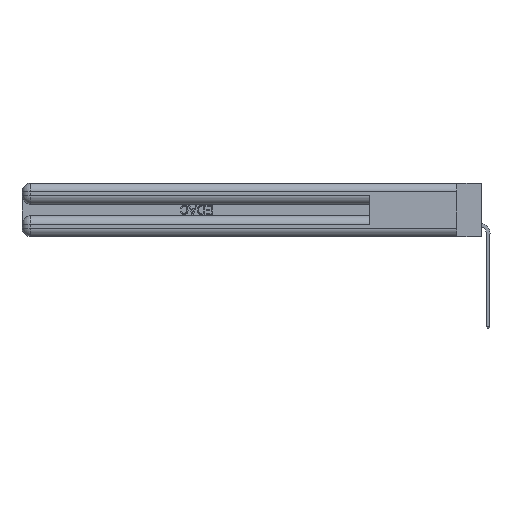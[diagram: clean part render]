
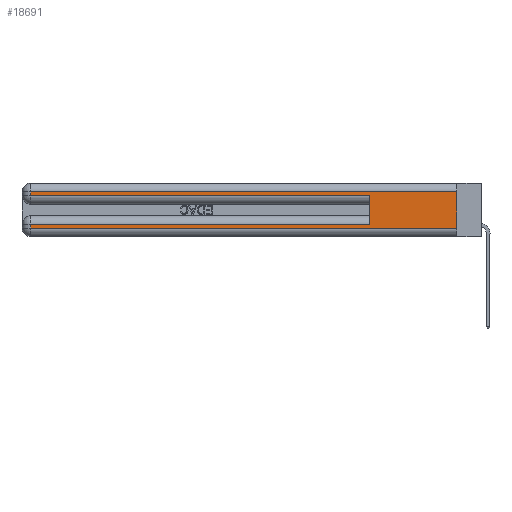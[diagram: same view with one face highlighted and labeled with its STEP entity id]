
A CAD part, left-side view. The second image highlights one B-rep face of the part: STEP entity #18691.
In plain terms, the highlighted planar face has unit normal (-1, 0, 0).
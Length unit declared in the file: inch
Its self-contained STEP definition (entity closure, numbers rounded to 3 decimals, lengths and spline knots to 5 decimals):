
#253 = LINE ( 'NONE', #23787, #23761 ) ;
#607 = CARTESIAN_POINT ( 'NONE',  ( 0., 2.94, 0.285 ) ) ;
#919 = VERTEX_POINT ( 'NONE', #7942 ) ;
#1976 = EDGE_CURVE ( 'NONE', #4796, #17353, #26263, .T. ) ;
#2054 = PLANE ( 'NONE',  #35698 ) ;
#2507 = DIRECTION ( 'NONE',  ( 0., 0., -1. ) ) ;
#3326 = ORIENTED_EDGE ( 'NONE', *, *, #7825, .T. ) ;
#3944 = EDGE_CURVE ( 'NONE', #32960, #919, #253, .T. ) ;
#4224 = LINE ( 'NONE', #21751, #16475 ) ;
#4229 = VERTEX_POINT ( 'NONE', #607 ) ;
#4796 = VERTEX_POINT ( 'NONE', #25364 ) ;
#4893 = DIRECTION ( 'NONE',  ( 0., 1., 0. ) ) ;
#4977 = CARTESIAN_POINT ( 'NONE',  ( 0., 2.94, 0.31 ) ) ;
#5818 = LINE ( 'NONE', #26309, #6734 ) ;
#6442 = FACE_OUTER_BOUND ( 'NONE', #36569, .T. ) ;
#6734 = VECTOR ( 'NONE', #26450, 39.37008 ) ;
#6960 = ORIENTED_EDGE ( 'NONE', *, *, #1976, .T. ) ;
#7302 = EDGE_CURVE ( 'NONE', #8050, #24421, #7932, .T. ) ;
#7433 = LINE ( 'NONE', #16743, #38401 ) ;
#7460 = VECTOR ( 'NONE', #38694, 39.37008 ) ;
#7825 = EDGE_CURVE ( 'NONE', #8050, #9718, #7433, .T. ) ;
#7852 = DIRECTION ( 'NONE',  ( 0., -1., 0. ) ) ;
#7881 = ORIENTED_EDGE ( 'NONE', *, *, #24158, .T. ) ;
#7932 = LINE ( 'NONE', #17477, #25278 ) ;
#7942 = CARTESIAN_POINT ( 'NONE',  ( 0., 0.6, 0.285 ) ) ;
#8050 = VERTEX_POINT ( 'NONE', #26896 ) ;
#8939 = DIRECTION ( 'NONE',  ( 0., 0., 1. ) ) ;
#9718 = VERTEX_POINT ( 'NONE', #4977 ) ;
#9908 = VECTOR ( 'NONE', #12853, 39.37008 ) ;
#10352 = EDGE_CURVE ( 'NONE', #9718, #4229, #5818, .T. ) ;
#11019 = ORIENTED_EDGE ( 'NONE', *, *, #7302, .F. ) ;
#11066 = CARTESIAN_POINT ( 'NONE',  ( 0., 0., 0.06 ) ) ;
#11372 = ORIENTED_EDGE ( 'NONE', *, *, #3944, .F. ) ;
#12537 = DIRECTION ( 'NONE',  ( 0., 0., -1. ) ) ;
#12647 = ORIENTED_EDGE ( 'NONE', *, *, #10352, .T. ) ;
#12853 = DIRECTION ( 'NONE',  ( 0., -1., 0. ) ) ;
#13716 = LINE ( 'NONE', #16249, #9908 ) ;
#14641 = CARTESIAN_POINT ( 'NONE',  ( 0., 2.94, 0.37 ) ) ;
#14891 = ORIENTED_EDGE ( 'NONE', *, *, #37552, .T. ) ;
#15171 = CARTESIAN_POINT ( 'NONE',  ( 0., 0., 0.37 ) ) ;
#16249 = CARTESIAN_POINT ( 'NONE',  ( 0., 0., 0.285 ) ) ;
#16475 = VECTOR ( 'NONE', #34582, 39.37008 ) ;
#16559 = CARTESIAN_POINT ( 'NONE',  ( 0., 0.6, 0.085 ) ) ;
#16743 = CARTESIAN_POINT ( 'NONE',  ( 0., 0., 0.31 ) ) ;
#16807 = CARTESIAN_POINT ( 'NONE',  ( 0., 0., 0.06 ) ) ;
#17224 = ORIENTED_EDGE ( 'NONE', *, *, #22716, .T. ) ;
#17353 = VERTEX_POINT ( 'NONE', #18235 ) ;
#17477 = CARTESIAN_POINT ( 'NONE',  ( 0., 0., 0.37 ) ) ;
#18235 = CARTESIAN_POINT ( 'NONE',  ( 0., 2.94, 0.06 ) ) ;
#18548 = DIRECTION ( 'NONE',  ( 1., 0., 0. ) ) ;
#18691 = ADVANCED_FACE ( 'NONE', ( #6442 ), #2054, .F. ) ;
#19853 = VECTOR ( 'NONE', #7852, 39.37008 ) ;
#21751 = CARTESIAN_POINT ( 'NONE',  ( 0., 0., 0.085 ) ) ;
#22716 = EDGE_CURVE ( 'NONE', #17353, #24421, #28770, .T. ) ;
#23761 = VECTOR ( 'NONE', #8939, 39.37008 ) ;
#23787 = CARTESIAN_POINT ( 'NONE',  ( 0., 0.6, 0.145 ) ) ;
#24158 = EDGE_CURVE ( 'NONE', #4229, #919, #13716, .T. ) ;
#24421 = VERTEX_POINT ( 'NONE', #11066 ) ;
#25278 = VECTOR ( 'NONE', #2507, 39.37008 ) ;
#25364 = CARTESIAN_POINT ( 'NONE',  ( 0., 2.94, 0.085 ) ) ;
#26263 = LINE ( 'NONE', #14641, #7460 ) ;
#26309 = CARTESIAN_POINT ( 'NONE',  ( 0., 2.94, 0.37 ) ) ;
#26450 = DIRECTION ( 'NONE',  ( 0., 0., -1. ) ) ;
#26896 = CARTESIAN_POINT ( 'NONE',  ( 0., 0., 0.31 ) ) ;
#28770 = LINE ( 'NONE', #16807, #19853 ) ;
#32960 = VERTEX_POINT ( 'NONE', #16559 ) ;
#34582 = DIRECTION ( 'NONE',  ( 0., 1., 0. ) ) ;
#35698 = AXIS2_PLACEMENT_3D ( 'NONE', #15171, #18548, #12537 ) ;
#36569 = EDGE_LOOP ( 'NONE', ( #11019, #3326, #12647, #7881, #11372, #14891, #6960, #17224 ) ) ;
#37552 = EDGE_CURVE ( 'NONE', #32960, #4796, #4224, .T. ) ;
#38401 = VECTOR ( 'NONE', #4893, 39.37008 ) ;
#38694 = DIRECTION ( 'NONE',  ( 0., 0., -1. ) ) ;
